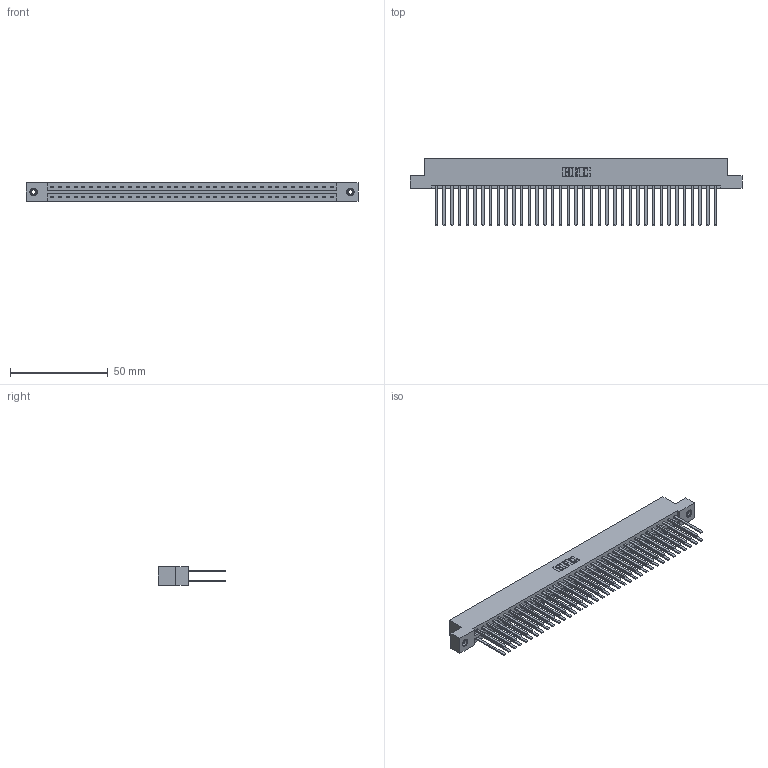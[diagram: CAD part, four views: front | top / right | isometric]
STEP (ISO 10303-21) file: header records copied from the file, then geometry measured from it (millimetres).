
FILE_DESCRIPTION (( 'STEP AP203' ), '1' );
FILE_NAME ('387-074-544-208.STEP', '2018-09-22T20:08:09', ( '' ), ( '' ), 'SwSTEP 2.0', 'SolidWorks 2016', '' );
FILE_SCHEMA (( 'CONFIG_CONTROL_DESIGN' ));
Length unit declared in the file: inch
Products named in the file (4): 337 Part_Flush Mounting Lugs - 0.156 Dia-TI; 345-292-001_345-293-144; 345-250-001_345-250-003-102; 387-074-544-208
Assembly tree (77 placements, depth 2):
  387-074-544-208
    337 Part_Flush Mounting Lugs - 0.156 Dia-TI
    345-292-001_345-293-144  x74
    345-250-001_345-250-003-102  x2
Bounding box: 169.62 x 34.3 x 9.4 mm (x, y, z)
Volume: 18840.3 mm3; surface area: 24663.1 mm2
Topology: 77 solids, 77 shells, 3726 faces, 11029 edges, 7246 vertices
Faces by surface type: plane 2618, cylinder 1092, cone 12, torus 4
Entity records: 30336 total; most frequent: CARTESIAN_POINT 5093, ORIENTED_EDGE 5022, DIRECTION 4369, EDGE_CURVE 2511, LINE 2367, VECTOR 2367, VERTEX_POINT 1668, AXIS2_PLACEMENT_3D 1001
